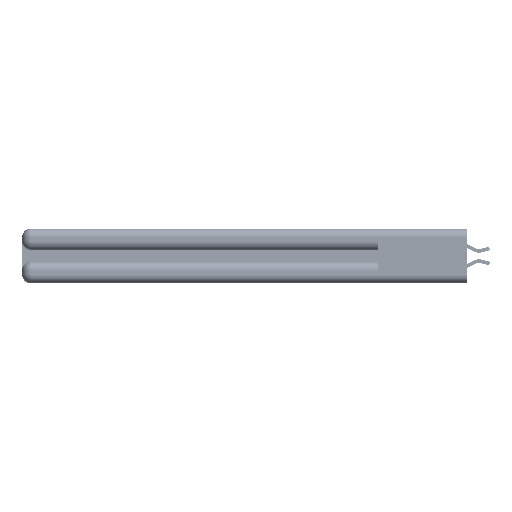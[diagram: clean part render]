
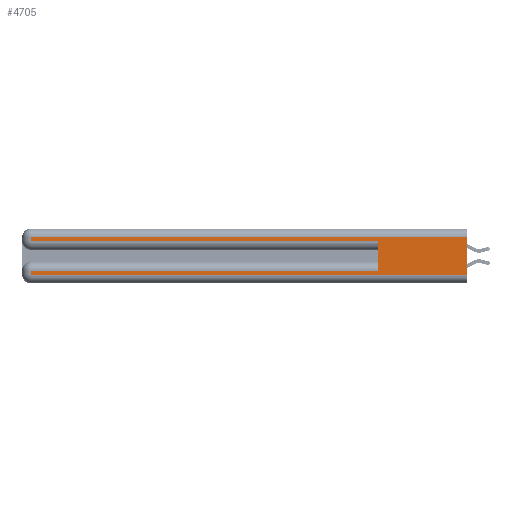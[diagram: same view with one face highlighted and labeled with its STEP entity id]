
A CAD part, left-side view. The second image highlights one B-rep face of the part: STEP entity #4705.
In plain terms, the highlighted planar face has unit normal (-1, 0, 0).
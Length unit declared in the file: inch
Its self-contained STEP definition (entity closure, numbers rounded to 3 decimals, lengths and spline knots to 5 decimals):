
#1192 = FACE_OUTER_BOUND ( 'NONE', #46731, .T. ) ;
#1904 = LINE ( 'NONE', #20230, #18031 ) ;
#1944 = DIRECTION ( 'NONE',  ( 0., 0., -1. ) ) ;
#1946 = CARTESIAN_POINT ( 'NONE',  ( 0., 2.94, 0.37 ) ) ;
#2033 = PLANE ( 'NONE',  #39889 ) ;
#2776 = ORIENTED_EDGE ( 'NONE', *, *, #29713, .T. ) ;
#3989 = DIRECTION ( 'NONE',  ( 0., -1., 0. ) ) ;
#4705 = ADVANCED_FACE ( 'NONE', ( #1192 ), #2033, .F. ) ;
#4808 = ORIENTED_EDGE ( 'NONE', *, *, #42079, .T. ) ;
#5809 = CARTESIAN_POINT ( 'NONE',  ( 0., 2.94, 0.085 ) ) ;
#6025 = DIRECTION ( 'NONE',  ( 1., 0., 0. ) ) ;
#6054 = LINE ( 'NONE', #26964, #7264 ) ;
#7205 = LINE ( 'NONE', #14346, #26354 ) ;
#7264 = VECTOR ( 'NONE', #41952, 39.37008 ) ;
#7366 = VERTEX_POINT ( 'NONE', #17768 ) ;
#7995 = CARTESIAN_POINT ( 'NONE',  ( 0., 0., 0.285 ) ) ;
#11023 = CARTESIAN_POINT ( 'NONE',  ( 0., 0., 0.06 ) ) ;
#11465 = CARTESIAN_POINT ( 'NONE',  ( 0., 0.6, 0.085 ) ) ;
#12579 = DIRECTION ( 'NONE',  ( 0., 0., -1. ) ) ;
#13505 = LINE ( 'NONE', #7995, #35548 ) ;
#13808 = VERTEX_POINT ( 'NONE', #47882 ) ;
#14346 = CARTESIAN_POINT ( 'NONE',  ( 0., 0., 0.06 ) ) ;
#14695 = EDGE_CURVE ( 'NONE', #48028, #27734, #7205, .T. ) ;
#14700 = CARTESIAN_POINT ( 'NONE',  ( 0., 0., 0.085 ) ) ;
#15825 = ORIENTED_EDGE ( 'NONE', *, *, #45804, .F. ) ;
#16340 = LINE ( 'NONE', #14700, #22876 ) ;
#17293 = LINE ( 'NONE', #38160, #34588 ) ;
#17768 = CARTESIAN_POINT ( 'NONE',  ( 0., 0., 0.31 ) ) ;
#18031 = VECTOR ( 'NONE', #12579, 39.37008 ) ;
#18154 = DIRECTION ( 'NONE',  ( 0., -1., 0. ) ) ;
#19365 = LINE ( 'NONE', #20791, #48604 ) ;
#20230 = CARTESIAN_POINT ( 'NONE',  ( 0., 2.94, 0.37 ) ) ;
#20791 = CARTESIAN_POINT ( 'NONE',  ( 0., 0., 0.37 ) ) ;
#22876 = VECTOR ( 'NONE', #41354, 39.37008 ) ;
#23223 = ORIENTED_EDGE ( 'NONE', *, *, #44743, .T. ) ;
#25415 = ORIENTED_EDGE ( 'NONE', *, *, #27353, .T. ) ;
#25476 = EDGE_CURVE ( 'NONE', #13808, #39615, #13505, .T. ) ;
#26354 = VECTOR ( 'NONE', #18154, 39.37008 ) ;
#26964 = CARTESIAN_POINT ( 'NONE',  ( 0., 0., 0.31 ) ) ;
#27002 = CARTESIAN_POINT ( 'NONE',  ( 0., 2.94, 0.31 ) ) ;
#27353 = EDGE_CURVE ( 'NONE', #31251, #13808, #1904, .T. ) ;
#27734 = VERTEX_POINT ( 'NONE', #11023 ) ;
#28051 = CARTESIAN_POINT ( 'NONE',  ( 0., 0.6, 0.285 ) ) ;
#28639 = DIRECTION ( 'NONE',  ( 0., 0., -1. ) ) ;
#28712 = CARTESIAN_POINT ( 'NONE',  ( 0., 0., 0.37 ) ) ;
#29195 = LINE ( 'NONE', #1946, #41056 ) ;
#29713 = EDGE_CURVE ( 'NONE', #40419, #48028, #29195, .T. ) ;
#31251 = VERTEX_POINT ( 'NONE', #27002 ) ;
#34588 = VECTOR ( 'NONE', #38482, 39.37008 ) ;
#35548 = VECTOR ( 'NONE', #3989, 39.37008 ) ;
#36645 = VERTEX_POINT ( 'NONE', #11465 ) ;
#38160 = CARTESIAN_POINT ( 'NONE',  ( 0., 0.6, 0.145 ) ) ;
#38482 = DIRECTION ( 'NONE',  ( 0., 0., 1. ) ) ;
#39615 = VERTEX_POINT ( 'NONE', #28051 ) ;
#39889 = AXIS2_PLACEMENT_3D ( 'NONE', #28712, #6025, #48380 ) ;
#40419 = VERTEX_POINT ( 'NONE', #5809 ) ;
#40990 = ORIENTED_EDGE ( 'NONE', *, *, #42650, .F. ) ;
#41056 = VECTOR ( 'NONE', #28639, 39.37008 ) ;
#41354 = DIRECTION ( 'NONE',  ( 0., 1., 0. ) ) ;
#41952 = DIRECTION ( 'NONE',  ( 0., 1., 0. ) ) ;
#42079 = EDGE_CURVE ( 'NONE', #36645, #40419, #16340, .T. ) ;
#42650 = EDGE_CURVE ( 'NONE', #7366, #27734, #19365, .T. ) ;
#43956 = ORIENTED_EDGE ( 'NONE', *, *, #14695, .T. ) ;
#44743 = EDGE_CURVE ( 'NONE', #7366, #31251, #6054, .T. ) ;
#44770 = CARTESIAN_POINT ( 'NONE',  ( 0., 2.94, 0.06 ) ) ;
#45804 = EDGE_CURVE ( 'NONE', #36645, #39615, #17293, .T. ) ;
#46611 = ORIENTED_EDGE ( 'NONE', *, *, #25476, .T. ) ;
#46731 = EDGE_LOOP ( 'NONE', ( #40990, #23223, #25415, #46611, #15825, #4808, #2776, #43956 ) ) ;
#47882 = CARTESIAN_POINT ( 'NONE',  ( 0., 2.94, 0.285 ) ) ;
#48028 = VERTEX_POINT ( 'NONE', #44770 ) ;
#48380 = DIRECTION ( 'NONE',  ( 0., 0., -1. ) ) ;
#48604 = VECTOR ( 'NONE', #1944, 39.37008 ) ;
